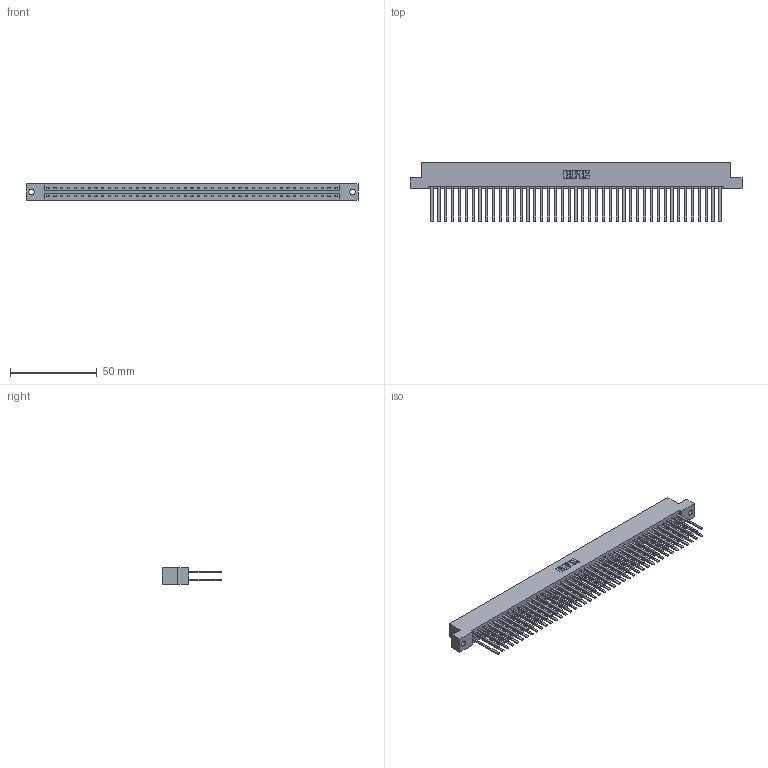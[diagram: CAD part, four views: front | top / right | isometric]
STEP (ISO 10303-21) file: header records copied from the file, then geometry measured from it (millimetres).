
FILE_DESCRIPTION (( 'STEP AP203' ), '1' );
FILE_NAME ('333-086-544-202.STEP', '2018-08-05T06:28:35', ( '' ), ( '' ), 'SwSTEP 2.0', 'SolidWorks 2016', '' );
FILE_SCHEMA (( 'CONFIG_CONTROL_DESIGN' ));
Length unit declared in the file: inch
Products named in the file (3): 333 Part_Flush - .128 Dia; 345-292-001_345-293-144; 333-086-544-202
Assembly tree (87 placements, depth 2):
  333-086-544-202
    333 Part_Flush - .128 Dia
    345-292-001_345-293-144  x86
Bounding box: 191.92 x 34.3 x 9.4 mm (x, y, z)
Volume: 20772.4 mm3; surface area: 28177.2 mm2
Topology: 87 solids, 87 shells, 4070 faces, 12093 edges, 7946 vertices
Faces by surface type: plane 2822, cylinder 1248
Entity records: 27353 total; most frequent: CARTESIAN_POINT 4530, ORIENTED_EDGE 4466, DIRECTION 3865, EDGE_CURVE 2233, LINE 2109, VECTOR 2109, VERTEX_POINT 1486, AXIS2_PLACEMENT_3D 878
